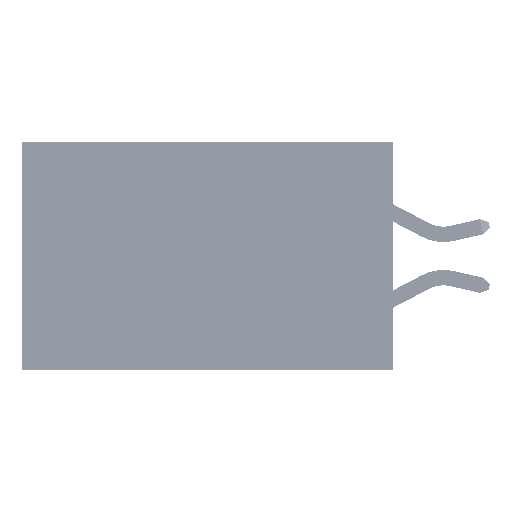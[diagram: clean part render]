
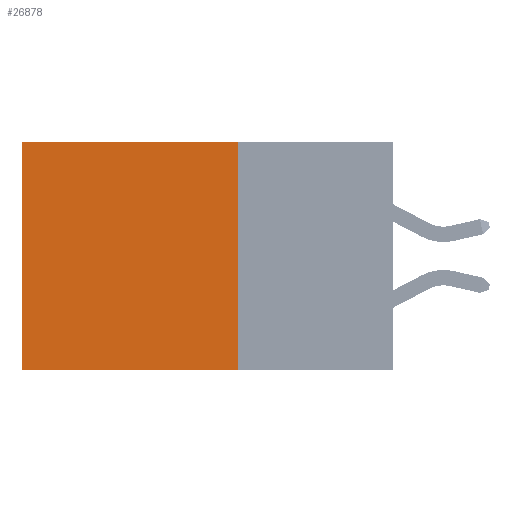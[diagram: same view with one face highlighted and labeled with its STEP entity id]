
A CAD part, left-side view. The second image highlights one B-rep face of the part: STEP entity #26878.
In plain terms, the highlighted planar face has unit normal (-1, 0, 0).
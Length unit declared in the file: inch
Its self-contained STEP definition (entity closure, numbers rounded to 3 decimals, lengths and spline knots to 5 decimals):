
#1028 = CARTESIAN_POINT ( 'NONE',  ( 0.2875, 0.25, 0. ) ) ;
#1178 = CARTESIAN_POINT ( 'NONE',  ( 0.2875, 0.25, 0. ) ) ;
#4382 = ORIENTED_EDGE ( 'NONE', *, *, #48818, .F. ) ;
#4544 = CARTESIAN_POINT ( 'NONE',  ( 0.2875, 0.25, 0. ) ) ;
#4983 = VERTEX_POINT ( 'NONE', #4544 ) ;
#6218 = EDGE_CURVE ( 'NONE', #4983, #46614, #11261, .T. ) ;
#6575 = AXIS2_PLACEMENT_3D ( 'NONE', #12796, #8318, #44143 ) ;
#8318 = DIRECTION ( 'NONE',  ( 1., 0., 0. ) ) ;
#8878 = VERTEX_POINT ( 'NONE', #14423 ) ;
#8883 = ORIENTED_EDGE ( 'NONE', *, *, #44222, .T. ) ;
#9583 = ORIENTED_EDGE ( 'NONE', *, *, #6218, .T. ) ;
#11261 = LINE ( 'NONE', #1178, #40737 ) ;
#12796 = CARTESIAN_POINT ( 'NONE',  ( 0.2875, 0.25, 0. ) ) ;
#14423 = CARTESIAN_POINT ( 'NONE',  ( 0.2875, 0.25, -0.37 ) ) ;
#16194 = VECTOR ( 'NONE', #28957, 39.37008 ) ;
#18531 = VECTOR ( 'NONE', #44047, 39.37008 ) ;
#21138 = LINE ( 'NONE', #25874, #16194 ) ;
#23128 = VERTEX_POINT ( 'NONE', #48139 ) ;
#25011 = DIRECTION ( 'NONE',  ( 0., 1., 0. ) ) ;
#25874 = CARTESIAN_POINT ( 'NONE',  ( 0.2875, 0.25, -0.37 ) ) ;
#26878 = ADVANCED_FACE ( 'NONE', ( #45646 ), #40025, .F. ) ;
#28957 = DIRECTION ( 'NONE',  ( 0., 1., 0. ) ) ;
#29587 = EDGE_LOOP ( 'NONE', ( #8883, #36382, #4382, #9583 ) ) ;
#31691 = CARTESIAN_POINT ( 'NONE',  ( 0.2875, 0.6, 0. ) ) ;
#35992 = EDGE_CURVE ( 'NONE', #8878, #23128, #21138, .T. ) ;
#36211 = VECTOR ( 'NONE', #42968, 39.37008 ) ;
#36382 = ORIENTED_EDGE ( 'NONE', *, *, #35992, .F. ) ;
#39227 = LINE ( 'NONE', #31691, #36211 ) ;
#40025 = PLANE ( 'NONE',  #6575 ) ;
#40737 = VECTOR ( 'NONE', #25011, 39.37008 ) ;
#42968 = DIRECTION ( 'NONE',  ( 0., 0., -1. ) ) ;
#44047 = DIRECTION ( 'NONE',  ( 0., 0., -1. ) ) ;
#44143 = DIRECTION ( 'NONE',  ( 0., 0., -1. ) ) ;
#44222 = EDGE_CURVE ( 'NONE', #46614, #23128, #39227, .T. ) ;
#44307 = CARTESIAN_POINT ( 'NONE',  ( 0.2875, 0.6, 0. ) ) ;
#45646 = FACE_OUTER_BOUND ( 'NONE', #29587, .T. ) ;
#46614 = VERTEX_POINT ( 'NONE', #44307 ) ;
#46725 = LINE ( 'NONE', #1028, #18531 ) ;
#48139 = CARTESIAN_POINT ( 'NONE',  ( 0.2875, 0.6, -0.37 ) ) ;
#48818 = EDGE_CURVE ( 'NONE', #4983, #8878, #46725, .T. ) ;
